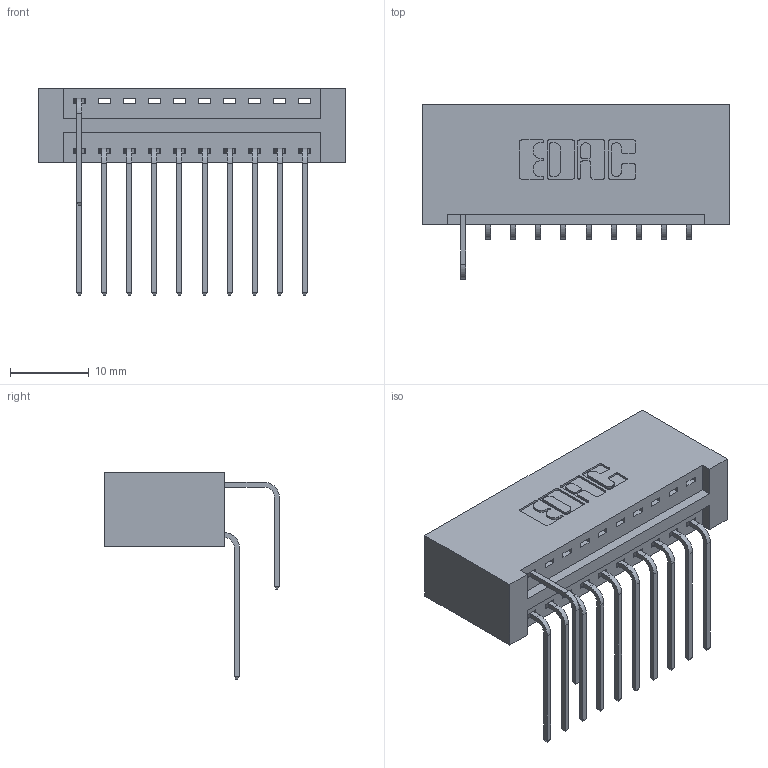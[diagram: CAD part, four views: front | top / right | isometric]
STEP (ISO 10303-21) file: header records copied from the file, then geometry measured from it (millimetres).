
FILE_DESCRIPTION (( 'STEP AP203' ), '1' );
FILE_NAME ('346-020-558-201.STEP', '2018-08-20T22:06:12', ( '' ), ( '' ), 'SwSTEP 2.0', 'SolidWorks 2016', '' );
FILE_SCHEMA (( 'CONFIG_CONTROL_DESIGN' ));
Length unit declared in the file: inch
Products named in the file (4): 346 Part_No Mounting Lugs; 345-292-001_558 559 Tail - 1; 345-292-001_558 Tail - 2; 346-020-558-201
Assembly tree (12 placements, depth 2):
  346-020-558-201
    346 Part_No Mounting Lugs
    345-292-001_558 559 Tail - 1  x10
    345-292-001_558 Tail - 2
Bounding box: 38.99 x 22.16 x 26.16 mm (x, y, z)
Volume: 4109.1 mm3; surface area: 5145.9 mm2
Topology: 12 solids, 12 shells, 762 faces, 2265 edges, 1494 vertices
Faces by surface type: plane 524, cylinder 238
Entity records: 12053 total; most frequent: CARTESIAN_POINT 2118, ORIENTED_EDGE 2010, DIRECTION 1875, EDGE_CURVE 1005, VECTOR 801, LINE 801, VERTEX_POINT 666, AXIS2_PLACEMENT_3D 537
